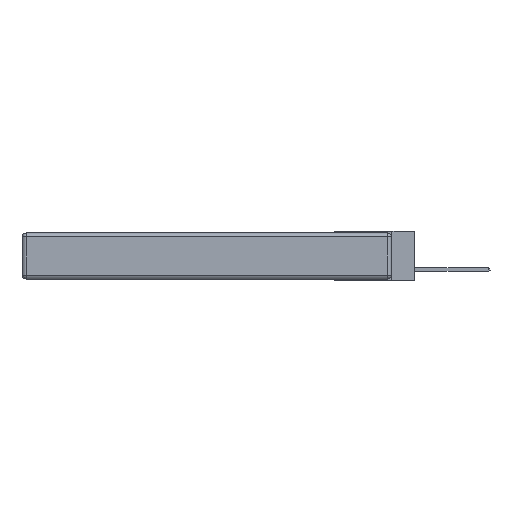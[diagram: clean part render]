
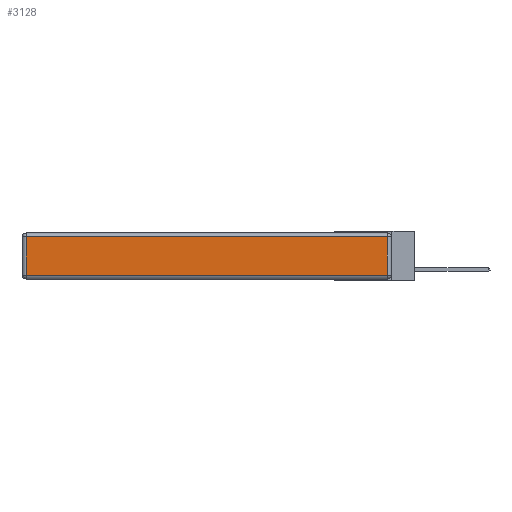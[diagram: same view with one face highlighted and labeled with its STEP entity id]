
A CAD part, left-side view. The second image highlights one B-rep face of the part: STEP entity #3128.
In plain terms, the highlighted planar face has unit normal (-1, 0, 0).
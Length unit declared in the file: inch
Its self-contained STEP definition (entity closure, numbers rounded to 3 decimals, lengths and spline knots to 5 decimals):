
#46 = VERTEX_POINT ( 'NONE', #11455 ) ;
#108 = EDGE_CURVE ( 'NONE', #46, #2819, #24132, .T. ) ;
#532 = CARTESIAN_POINT ( 'NONE',  ( 0., 2.72, -0.343 ) ) ;
#1412 = DIRECTION ( 'NONE',  ( 0., 0., 1. ) ) ;
#2013 = VECTOR ( 'NONE', #3835, 39.37008 ) ;
#2528 = LINE ( 'NONE', #16088, #21951 ) ;
#2819 = VERTEX_POINT ( 'NONE', #11064 ) ;
#3128 = ADVANCED_FACE ( 'NONE', ( #13150 ), #20391, .T. ) ;
#3175 = EDGE_LOOP ( 'NONE', ( #21497, #4544, #12583, #5914 ) ) ;
#3835 = DIRECTION ( 'NONE',  ( 0., 0., 1. ) ) ;
#4321 = DIRECTION ( 'NONE',  ( 0., 0., -1. ) ) ;
#4544 = ORIENTED_EDGE ( 'NONE', *, *, #5593, .T. ) ;
#4854 = DIRECTION ( 'NONE',  ( 0., -1., 0. ) ) ;
#5593 = EDGE_CURVE ( 'NONE', #21243, #46, #8501, .T. ) ;
#5683 = LINE ( 'NONE', #532, #8056 ) ;
#5914 = ORIENTED_EDGE ( 'NONE', *, *, #14755, .T. ) ;
#8056 = VECTOR ( 'NONE', #4321, 39.37008 ) ;
#8501 = LINE ( 'NONE', #13374, #2013 ) ;
#11064 = CARTESIAN_POINT ( 'NONE',  ( 0., 2.72, -0.03 ) ) ;
#11076 = VERTEX_POINT ( 'NONE', #19252 ) ;
#11455 = CARTESIAN_POINT ( 'NONE',  ( 0., 0.03, -0.03 ) ) ;
#12583 = ORIENTED_EDGE ( 'NONE', *, *, #108, .T. ) ;
#13150 = FACE_OUTER_BOUND ( 'NONE', #3175, .T. ) ;
#13374 = CARTESIAN_POINT ( 'NONE',  ( 0., 0.03, -0.343 ) ) ;
#14486 = AXIS2_PLACEMENT_3D ( 'NONE', #20469, #20312, #1412 ) ;
#14755 = EDGE_CURVE ( 'NONE', #2819, #11076, #5683, .T. ) ;
#16088 = CARTESIAN_POINT ( 'NONE',  ( 0., 0., -0.313 ) ) ;
#17245 = DIRECTION ( 'NONE',  ( 0., 1., 0. ) ) ;
#17366 = VECTOR ( 'NONE', #17245, 39.37008 ) ;
#18269 = CARTESIAN_POINT ( 'NONE',  ( 0., 0.03, -0.313 ) ) ;
#19252 = CARTESIAN_POINT ( 'NONE',  ( 0., 2.72, -0.313 ) ) ;
#20312 = DIRECTION ( 'NONE',  ( -1., 0., 0. ) ) ;
#20391 = PLANE ( 'NONE',  #14486 ) ;
#20469 = CARTESIAN_POINT ( 'NONE',  ( 0., 0., -0.343 ) ) ;
#21188 = CARTESIAN_POINT ( 'NONE',  ( 0., 2.75, -0.03 ) ) ;
#21243 = VERTEX_POINT ( 'NONE', #18269 ) ;
#21497 = ORIENTED_EDGE ( 'NONE', *, *, #23473, .T. ) ;
#21951 = VECTOR ( 'NONE', #4854, 39.37008 ) ;
#23473 = EDGE_CURVE ( 'NONE', #11076, #21243, #2528, .T. ) ;
#24132 = LINE ( 'NONE', #21188, #17366 ) ;
